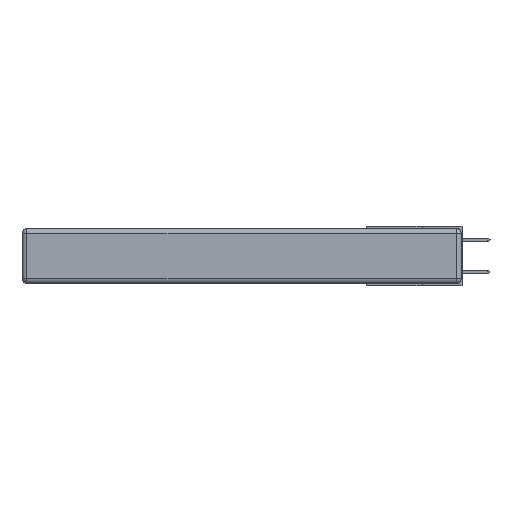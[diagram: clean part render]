
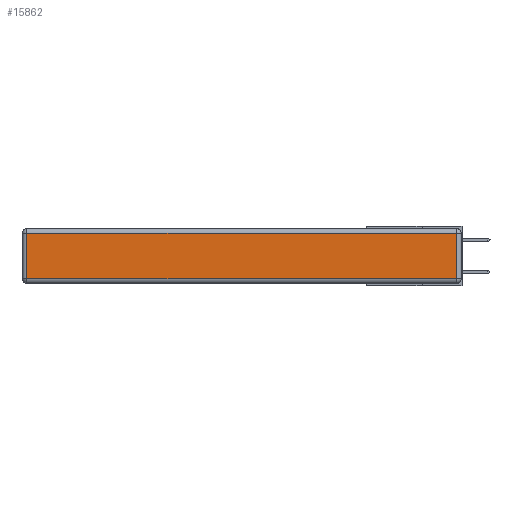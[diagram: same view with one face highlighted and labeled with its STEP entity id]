
A CAD part, left-side view. The second image highlights one B-rep face of the part: STEP entity #15862.
In plain terms, the highlighted planar face has unit normal (-1, 0, 0).
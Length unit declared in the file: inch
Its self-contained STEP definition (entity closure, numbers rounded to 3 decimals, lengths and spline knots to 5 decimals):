
#1029 = DIRECTION ( 'NONE',  ( 0., 0., 1. ) ) ;
#1699 = LINE ( 'NONE', #5899, #30472 ) ;
#2302 = CARTESIAN_POINT ( 'NONE',  ( 0., 2.72, -0.313 ) ) ;
#2662 = ORIENTED_EDGE ( 'NONE', *, *, #9017, .T. ) ;
#3655 = PLANE ( 'NONE',  #15146 ) ;
#3763 = VERTEX_POINT ( 'NONE', #2302 ) ;
#4292 = FACE_OUTER_BOUND ( 'NONE', #35590, .T. ) ;
#4489 = VERTEX_POINT ( 'NONE', #14384 ) ;
#4614 = CARTESIAN_POINT ( 'NONE',  ( 0., 0., -0.313 ) ) ;
#5120 = VERTEX_POINT ( 'NONE', #13207 ) ;
#5899 = CARTESIAN_POINT ( 'NONE',  ( 0., 0.03, -0.343 ) ) ;
#7301 = ORIENTED_EDGE ( 'NONE', *, *, #27101, .T. ) ;
#9017 = EDGE_CURVE ( 'NONE', #3763, #5120, #9166, .T. ) ;
#9166 = LINE ( 'NONE', #4614, #32344 ) ;
#11470 = EDGE_CURVE ( 'NONE', #4489, #3763, #23471, .T. ) ;
#11660 = ORIENTED_EDGE ( 'NONE', *, *, #23270, .T. ) ;
#12397 = VERTEX_POINT ( 'NONE', #15660 ) ;
#13207 = CARTESIAN_POINT ( 'NONE',  ( 0., 0.03, -0.313 ) ) ;
#14342 = DIRECTION ( 'NONE',  ( 0., 1., 0. ) ) ;
#14384 = CARTESIAN_POINT ( 'NONE',  ( 0., 2.72, -0.03 ) ) ;
#14768 = CARTESIAN_POINT ( 'NONE',  ( 0., 2.72, -0.343 ) ) ;
#15146 = AXIS2_PLACEMENT_3D ( 'NONE', #31568, #32427, #15232 ) ;
#15232 = DIRECTION ( 'NONE',  ( 0., 0., 1. ) ) ;
#15660 = CARTESIAN_POINT ( 'NONE',  ( 0., 0.03, -0.03 ) ) ;
#15862 = ADVANCED_FACE ( 'NONE', ( #4292 ), #3655, .T. ) ;
#17709 = DIRECTION ( 'NONE',  ( 0., 0., -1. ) ) ;
#19033 = LINE ( 'NONE', #21913, #32579 ) ;
#21913 = CARTESIAN_POINT ( 'NONE',  ( 0., 2.75, -0.03 ) ) ;
#23204 = ORIENTED_EDGE ( 'NONE', *, *, #11470, .T. ) ;
#23270 = EDGE_CURVE ( 'NONE', #12397, #4489, #19033, .T. ) ;
#23471 = LINE ( 'NONE', #14768, #32209 ) ;
#27101 = EDGE_CURVE ( 'NONE', #5120, #12397, #1699, .T. ) ;
#30472 = VECTOR ( 'NONE', #1029, 39.37008 ) ;
#31568 = CARTESIAN_POINT ( 'NONE',  ( 0., 0., -0.343 ) ) ;
#32209 = VECTOR ( 'NONE', #17709, 39.37008 ) ;
#32344 = VECTOR ( 'NONE', #35350, 39.37008 ) ;
#32427 = DIRECTION ( 'NONE',  ( -1., 0., 0. ) ) ;
#32579 = VECTOR ( 'NONE', #14342, 39.37008 ) ;
#35350 = DIRECTION ( 'NONE',  ( 0., -1., 0. ) ) ;
#35590 = EDGE_LOOP ( 'NONE', ( #2662, #7301, #11660, #23204 ) ) ;
